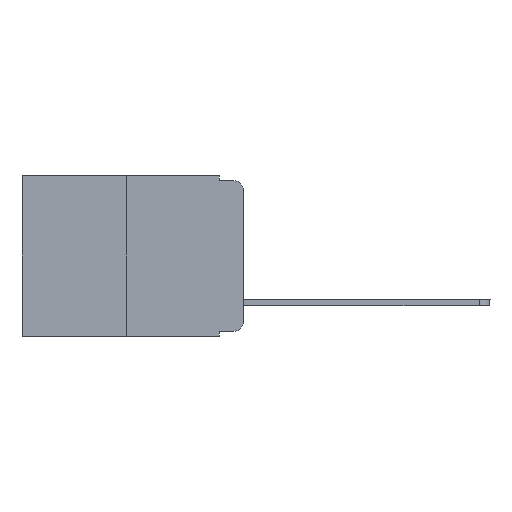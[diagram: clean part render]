
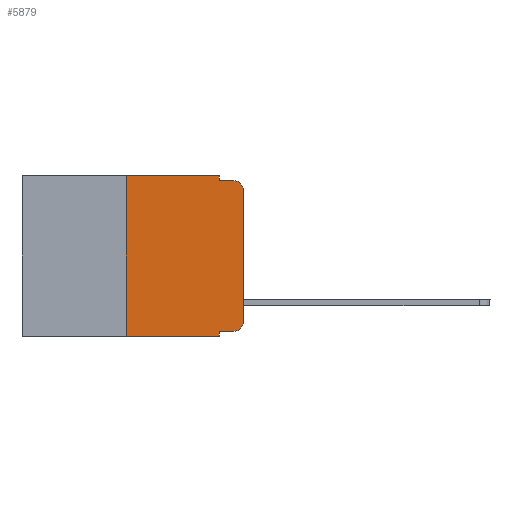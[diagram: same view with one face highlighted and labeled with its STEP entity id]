
A CAD part, left-side view. The second image highlights one B-rep face of the part: STEP entity #5879.
In plain terms, the highlighted planar face has unit normal (-1, 0, 0).
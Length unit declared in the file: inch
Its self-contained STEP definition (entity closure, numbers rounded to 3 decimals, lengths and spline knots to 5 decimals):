
#100 = VECTOR ( 'NONE', #8246, 39.37008 ) ;
#489 = VECTOR ( 'NONE', #1328, 39.37008 ) ;
#500 = CARTESIAN_POINT ( 'NONE',  ( 0., 0.02, -0.333 ) ) ;
#594 = LINE ( 'NONE', #7726, #4058 ) ;
#928 = VERTEX_POINT ( 'NONE', #15286 ) ;
#1328 = DIRECTION ( 'NONE',  ( 0., -1., 0. ) ) ;
#1566 = ORIENTED_EDGE ( 'NONE', *, *, #16061, .T. ) ;
#1693 = CARTESIAN_POINT ( 'NONE',  ( 0., 0.02, -0.313 ) ) ;
#1964 = VECTOR ( 'NONE', #15324, 39.37008 ) ;
#1984 = EDGE_LOOP ( 'NONE', ( #10712, #1566, #10179, #15418, #9551, #17007, #3135, #9987, #8737, #14216 ) ) ;
#2395 = CARTESIAN_POINT ( 'NONE',  ( 0., 0.051, -0.01 ) ) ;
#2434 = VECTOR ( 'NONE', #9849, 39.37008 ) ;
#2740 = VECTOR ( 'NONE', #7525, 39.37008 ) ;
#2944 = CARTESIAN_POINT ( 'NONE',  ( 0., 0.051, 0. ) ) ;
#3122 = VERTEX_POINT ( 'NONE', #5577 ) ;
#3135 = ORIENTED_EDGE ( 'NONE', *, *, #13608, .T. ) ;
#3825 = DIRECTION ( 'NONE',  ( 0., 0., -1. ) ) ;
#3840 = LINE ( 'NONE', #9228, #15247 ) ;
#3989 = EDGE_CURVE ( 'NONE', #928, #16638, #8421, .T. ) ;
#4058 = VECTOR ( 'NONE', #14659, 39.37008 ) ;
#4126 = VERTEX_POINT ( 'NONE', #15924 ) ;
#4217 = LINE ( 'NONE', #16824, #15831 ) ;
#5577 = CARTESIAN_POINT ( 'NONE',  ( 0., 0.02, -0.01 ) ) ;
#5879 = ADVANCED_FACE ( 'NONE', ( #12214 ), #6576, .F. ) ;
#5998 = AXIS2_PLACEMENT_3D ( 'NONE', #12805, #11353, #8889 ) ;
#6160 = CARTESIAN_POINT ( 'NONE',  ( 0., 0.25, 0. ) ) ;
#6576 = PLANE ( 'NONE',  #16067 ) ;
#6632 = VERTEX_POINT ( 'NONE', #500 ) ;
#7525 = DIRECTION ( 'NONE',  ( 0., -1., 0. ) ) ;
#7726 = CARTESIAN_POINT ( 'NONE',  ( 0., 0.25, 0. ) ) ;
#7935 = EDGE_CURVE ( 'NONE', #15869, #15011, #594, .T. ) ;
#8110 = CARTESIAN_POINT ( 'NONE',  ( 0., 0.051, -0.343 ) ) ;
#8246 = DIRECTION ( 'NONE',  ( 0., 0., -1. ) ) ;
#8421 = LINE ( 'NONE', #2944, #100 ) ;
#8737 = ORIENTED_EDGE ( 'NONE', *, *, #12572, .T. ) ;
#8889 = DIRECTION ( 'NONE',  ( 0., 0., -1. ) ) ;
#9228 = CARTESIAN_POINT ( 'NONE',  ( 0., 0.473, -0.343 ) ) ;
#9255 = CARTESIAN_POINT ( 'NONE',  ( 0., 0.051, -0.01 ) ) ;
#9369 = EDGE_CURVE ( 'NONE', #15011, #928, #17785, .T. ) ;
#9551 = ORIENTED_EDGE ( 'NONE', *, *, #9369, .F. ) ;
#9849 = DIRECTION ( 'NONE',  ( 0., -1., 0. ) ) ;
#9899 = DIRECTION ( 'NONE',  ( 0., 0., -1. ) ) ;
#9917 = VERTEX_POINT ( 'NONE', #12110 ) ;
#9930 = LINE ( 'NONE', #15503, #1964 ) ;
#9987 = ORIENTED_EDGE ( 'NONE', *, *, #17420, .F. ) ;
#10179 = ORIENTED_EDGE ( 'NONE', *, *, #15037, .F. ) ;
#10712 = ORIENTED_EDGE ( 'NONE', *, *, #12063, .T. ) ;
#11197 = CIRCLE ( 'NONE', #13549, 0.02 ) ;
#11353 = DIRECTION ( 'NONE',  ( -1., 0., 0. ) ) ;
#11521 = CIRCLE ( 'NONE', #5998, 0.02 ) ;
#12063 = EDGE_CURVE ( 'NONE', #16325, #4126, #4217, .T. ) ;
#12081 = CARTESIAN_POINT ( 'NONE',  ( 0., 0., -0.313 ) ) ;
#12095 = CARTESIAN_POINT ( 'NONE',  ( 0., 0.473, 0. ) ) ;
#12110 = CARTESIAN_POINT ( 'NONE',  ( 0., 0.051, -0.333 ) ) ;
#12214 = FACE_OUTER_BOUND ( 'NONE', #1984, .T. ) ;
#12311 = LINE ( 'NONE', #15334, #2434 ) ;
#12332 = DIRECTION ( 'NONE',  ( 0., 0., 1. ) ) ;
#12572 = EDGE_CURVE ( 'NONE', #9917, #6632, #12311, .T. ) ;
#12805 = CARTESIAN_POINT ( 'NONE',  ( 0., 0.02, -0.03 ) ) ;
#13364 = LINE ( 'NONE', #9255, #2740 ) ;
#13482 = CARTESIAN_POINT ( 'NONE',  ( 0., 0.25, -0.343 ) ) ;
#13549 = AXIS2_PLACEMENT_3D ( 'NONE', #1693, #16859, #9899 ) ;
#13608 = EDGE_CURVE ( 'NONE', #15869, #14358, #3840, .T. ) ;
#13683 = CARTESIAN_POINT ( 'NONE',  ( 0., 0.473, 0. ) ) ;
#14216 = ORIENTED_EDGE ( 'NONE', *, *, #14864, .T. ) ;
#14358 = VERTEX_POINT ( 'NONE', #8110 ) ;
#14659 = DIRECTION ( 'NONE',  ( 0., 0., 1. ) ) ;
#14864 = EDGE_CURVE ( 'NONE', #6632, #16325, #11197, .T. ) ;
#14901 = DIRECTION ( 'NONE',  ( 0., -1., 0. ) ) ;
#15011 = VERTEX_POINT ( 'NONE', #6160 ) ;
#15037 = EDGE_CURVE ( 'NONE', #16638, #3122, #13364, .T. ) ;
#15247 = VECTOR ( 'NONE', #14901, 39.37008 ) ;
#15286 = CARTESIAN_POINT ( 'NONE',  ( 0., 0.051, 0. ) ) ;
#15324 = DIRECTION ( 'NONE',  ( 0., 0., -1. ) ) ;
#15334 = CARTESIAN_POINT ( 'NONE',  ( 0., 0.051, -0.333 ) ) ;
#15418 = ORIENTED_EDGE ( 'NONE', *, *, #3989, .F. ) ;
#15503 = CARTESIAN_POINT ( 'NONE',  ( 0., 0.051, 0. ) ) ;
#15831 = VECTOR ( 'NONE', #12332, 39.37008 ) ;
#15869 = VERTEX_POINT ( 'NONE', #13482 ) ;
#15924 = CARTESIAN_POINT ( 'NONE',  ( 0., 0., -0.03 ) ) ;
#16061 = EDGE_CURVE ( 'NONE', #4126, #3122, #11521, .T. ) ;
#16067 = AXIS2_PLACEMENT_3D ( 'NONE', #13683, #16350, #3825 ) ;
#16325 = VERTEX_POINT ( 'NONE', #12081 ) ;
#16350 = DIRECTION ( 'NONE',  ( 1., 0., 0. ) ) ;
#16638 = VERTEX_POINT ( 'NONE', #2395 ) ;
#16824 = CARTESIAN_POINT ( 'NONE',  ( 0., 0., 0. ) ) ;
#16859 = DIRECTION ( 'NONE',  ( -1., 0., 0. ) ) ;
#17007 = ORIENTED_EDGE ( 'NONE', *, *, #7935, .F. ) ;
#17420 = EDGE_CURVE ( 'NONE', #9917, #14358, #9930, .T. ) ;
#17785 = LINE ( 'NONE', #12095, #489 ) ;
